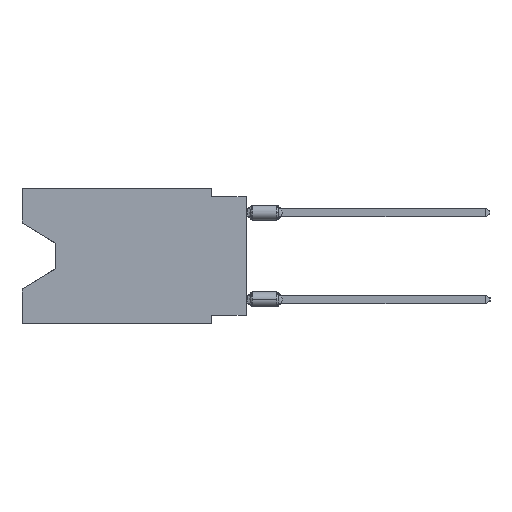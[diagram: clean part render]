
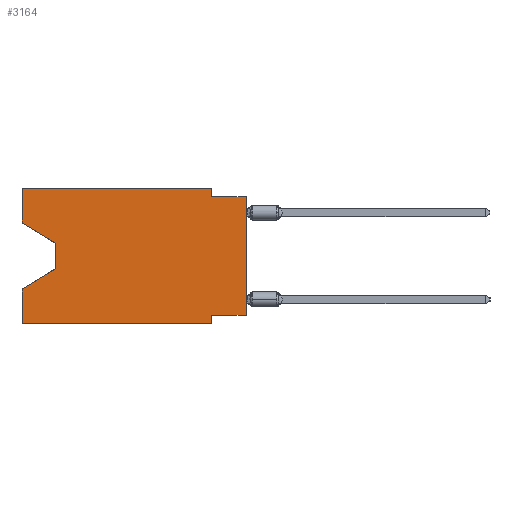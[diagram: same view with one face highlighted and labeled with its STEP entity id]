
A CAD part, left-side view. The second image highlights one B-rep face of the part: STEP entity #3164.
In plain terms, the highlighted planar face has unit normal (-1, 0, 0).
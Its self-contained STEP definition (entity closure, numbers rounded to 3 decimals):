
#362 = LINE ( 'NONE', #16299, #12759 ) ;
#996 = VECTOR ( 'NONE', #6829, 1000. ) ;
#1036 = EDGE_CURVE ( 'NONE', #19545, #2599, #7957, .T. ) ;
#1102 = EDGE_CURVE ( 'NONE', #25374, #13089, #4387, .T. ) ;
#1193 = VERTEX_POINT ( 'NONE', #33186 ) ;
#1488 = CARTESIAN_POINT ( 'NONE',  ( 0., 2.54, -9.906 ) ) ;
#1765 = CARTESIAN_POINT ( 'NONE',  ( 0., 0., -9.271 ) ) ;
#2457 = DIRECTION ( 'NONE',  ( 0., -1., 0. ) ) ;
#2599 = VERTEX_POINT ( 'NONE', #28152 ) ;
#2637 = CARTESIAN_POINT ( 'NONE',  ( 0., 16.383, -2.546 ) ) ;
#2707 = DIRECTION ( 'NONE',  ( 0., 0., 1. ) ) ;
#2761 = AXIS2_PLACEMENT_3D ( 'NONE', #25335, #3642, #22851 ) ;
#2845 = LINE ( 'NONE', #25065, #9519 ) ;
#3089 = EDGE_CURVE ( 'NONE', #30296, #22919, #11376, .T. ) ;
#3164 = ADVANCED_FACE ( 'NONE', ( #6334 ), #26046, .F. ) ;
#3642 = DIRECTION ( 'NONE',  ( 1., 0., 0. ) ) ;
#4119 = CARTESIAN_POINT ( 'NONE',  ( 0., 13.97, -4.013 ) ) ;
#4160 = LINE ( 'NONE', #1488, #12137 ) ;
#4387 = LINE ( 'NONE', #15313, #4440 ) ;
#4440 = VECTOR ( 'NONE', #15642, 1000. ) ;
#4961 = VERTEX_POINT ( 'NONE', #11040 ) ;
#4972 = CARTESIAN_POINT ( 'NONE',  ( 0., 0., -9.271 ) ) ;
#5000 = VECTOR ( 'NONE', #27335, 1000. ) ;
#5721 = ORIENTED_EDGE ( 'NONE', *, *, #3089, .F. ) ;
#6334 = FACE_OUTER_BOUND ( 'NONE', #12118, .T. ) ;
#6446 = LINE ( 'NONE', #4119, #996 ) ;
#6829 = DIRECTION ( 'NONE',  ( 0., 0., -1. ) ) ;
#6873 = CARTESIAN_POINT ( 'NONE',  ( 0., 16.383, -9.906 ) ) ;
#7672 = EDGE_CURVE ( 'NONE', #17370, #2599, #2845, .T. ) ;
#7696 = ORIENTED_EDGE ( 'NONE', *, *, #33910, .T. ) ;
#7957 = LINE ( 'NONE', #18183, #8455 ) ;
#8455 = VECTOR ( 'NONE', #21590, 1000. ) ;
#8662 = LINE ( 'NONE', #22466, #14407 ) ;
#8676 = VERTEX_POINT ( 'NONE', #26747 ) ;
#9167 = VERTEX_POINT ( 'NONE', #13416 ) ;
#9347 = DIRECTION ( 'NONE',  ( 0., 0., -1. ) ) ;
#9519 = VECTOR ( 'NONE', #16987, 1000. ) ;
#9590 = ORIENTED_EDGE ( 'NONE', *, *, #33284, .F. ) ;
#9968 = ORIENTED_EDGE ( 'NONE', *, *, #34132, .F. ) ;
#10337 = CARTESIAN_POINT ( 'NONE',  ( 0., 13.97, -4.013 ) ) ;
#10738 = ORIENTED_EDGE ( 'NONE', *, *, #7672, .T. ) ;
#10828 = ORIENTED_EDGE ( 'NONE', *, *, #1102, .T. ) ;
#11040 = CARTESIAN_POINT ( 'NONE',  ( 0., 2.54, -9.271 ) ) ;
#11376 = LINE ( 'NONE', #33212, #5000 ) ;
#11569 = LINE ( 'NONE', #17845, #12924 ) ;
#12118 = EDGE_LOOP ( 'NONE', ( #10828, #31901, #12370, #5721, #7696, #9968, #13815, #10738, #20544, #9590, #17397, #20548 ) ) ;
#12137 = VECTOR ( 'NONE', #9347, 1000. ) ;
#12184 = VECTOR ( 'NONE', #2707, 1000. ) ;
#12370 = ORIENTED_EDGE ( 'NONE', *, *, #31450, .T. ) ;
#12759 = VECTOR ( 'NONE', #30093, 1000. ) ;
#12924 = VECTOR ( 'NONE', #14432, 1000. ) ;
#13089 = VERTEX_POINT ( 'NONE', #10337 ) ;
#13140 = EDGE_CURVE ( 'NONE', #9167, #27185, #26835, .T. ) ;
#13416 = CARTESIAN_POINT ( 'NONE',  ( 0., 16.383, 0. ) ) ;
#13815 = ORIENTED_EDGE ( 'NONE', *, *, #28921, .F. ) ;
#14407 = VECTOR ( 'NONE', #2457, 1000. ) ;
#14432 = DIRECTION ( 'NONE',  ( 0., 0.855, -0.519 ) ) ;
#15313 = CARTESIAN_POINT ( 'NONE',  ( 0., 16.383, -2.546 ) ) ;
#15642 = DIRECTION ( 'NONE',  ( 0., -0.855, -0.519 ) ) ;
#16299 = CARTESIAN_POINT ( 'NONE',  ( 0., 2.54, 0. ) ) ;
#16987 = DIRECTION ( 'NONE',  ( 0., 0., 1. ) ) ;
#17370 = VERTEX_POINT ( 'NONE', #4972 ) ;
#17397 = ORIENTED_EDGE ( 'NONE', *, *, #13140, .F. ) ;
#17766 = CARTESIAN_POINT ( 'NONE',  ( 0., 16.383, -7.36 ) ) ;
#17845 = CARTESIAN_POINT ( 'NONE',  ( 0., 13.97, -5.893 ) ) ;
#18183 = CARTESIAN_POINT ( 'NONE',  ( 0., 0., -0.635 ) ) ;
#18949 = DIRECTION ( 'NONE',  ( 0., -1., 0. ) ) ;
#19545 = VERTEX_POINT ( 'NONE', #31068 ) ;
#20544 = ORIENTED_EDGE ( 'NONE', *, *, #1036, .F. ) ;
#20548 = ORIENTED_EDGE ( 'NONE', *, *, #33299, .F. ) ;
#21496 = VECTOR ( 'NONE', #31670, 1000. ) ;
#21590 = DIRECTION ( 'NONE',  ( 0., -1., 0. ) ) ;
#22466 = CARTESIAN_POINT ( 'NONE',  ( 0., 16.383, -9.906 ) ) ;
#22851 = DIRECTION ( 'NONE',  ( 0., 0., -1. ) ) ;
#22919 = VERTEX_POINT ( 'NONE', #17766 ) ;
#25065 = CARTESIAN_POINT ( 'NONE',  ( 0., 0., 0. ) ) ;
#25335 = CARTESIAN_POINT ( 'NONE',  ( 0., 16.383, 0. ) ) ;
#25374 = VERTEX_POINT ( 'NONE', #2637 ) ;
#26046 = PLANE ( 'NONE',  #2761 ) ;
#26479 = LINE ( 'NONE', #1765, #21496 ) ;
#26681 = CARTESIAN_POINT ( 'NONE',  ( 0., 2.54, 0. ) ) ;
#26747 = CARTESIAN_POINT ( 'NONE',  ( 0., 13.97, -5.893 ) ) ;
#26835 = LINE ( 'NONE', #29156, #34628 ) ;
#27185 = VERTEX_POINT ( 'NONE', #26681 ) ;
#27239 = LINE ( 'NONE', #32759, #12184 ) ;
#27335 = DIRECTION ( 'NONE',  ( 0., 0., 1. ) ) ;
#28152 = CARTESIAN_POINT ( 'NONE',  ( 0., 0., -0.635 ) ) ;
#28921 = EDGE_CURVE ( 'NONE', #17370, #4961, #26479, .T. ) ;
#29156 = CARTESIAN_POINT ( 'NONE',  ( 0., 16.383, 0. ) ) ;
#30093 = DIRECTION ( 'NONE',  ( 0., 0., -1. ) ) ;
#30296 = VERTEX_POINT ( 'NONE', #6873 ) ;
#31068 = CARTESIAN_POINT ( 'NONE',  ( 0., 2.54, -0.635 ) ) ;
#31450 = EDGE_CURVE ( 'NONE', #8676, #22919, #11569, .T. ) ;
#31670 = DIRECTION ( 'NONE',  ( 0., 1., 0. ) ) ;
#31901 = ORIENTED_EDGE ( 'NONE', *, *, #33047, .T. ) ;
#32759 = CARTESIAN_POINT ( 'NONE',  ( 0., 16.383, 0. ) ) ;
#33047 = EDGE_CURVE ( 'NONE', #13089, #8676, #6446, .T. ) ;
#33186 = CARTESIAN_POINT ( 'NONE',  ( 0., 2.54, -9.906 ) ) ;
#33212 = CARTESIAN_POINT ( 'NONE',  ( 0., 16.383, 0. ) ) ;
#33284 = EDGE_CURVE ( 'NONE', #27185, #19545, #362, .T. ) ;
#33299 = EDGE_CURVE ( 'NONE', #25374, #9167, #27239, .T. ) ;
#33910 = EDGE_CURVE ( 'NONE', #30296, #1193, #8662, .T. ) ;
#34132 = EDGE_CURVE ( 'NONE', #4961, #1193, #4160, .T. ) ;
#34628 = VECTOR ( 'NONE', #18949, 1000. ) ;
